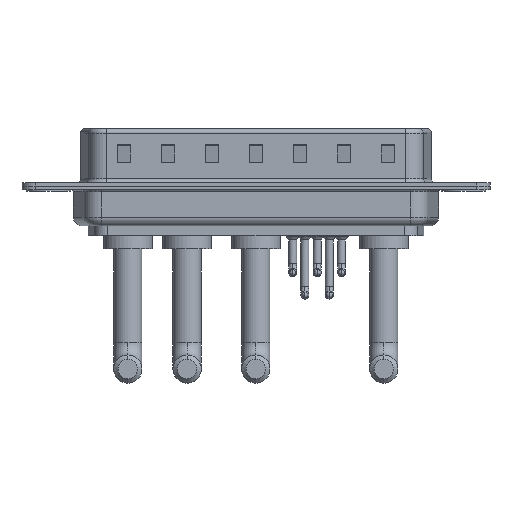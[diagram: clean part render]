
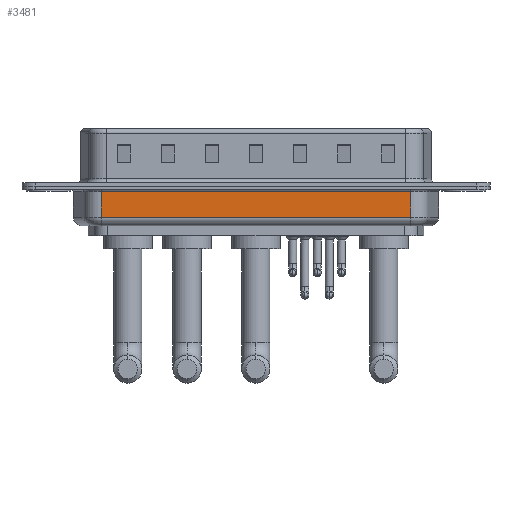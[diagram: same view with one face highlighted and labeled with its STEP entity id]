
A CAD part, front view. The second image highlights one B-rep face of the part: STEP entity #3481.
In plain terms, the highlighted planar face has unit normal (0, -1, 0).
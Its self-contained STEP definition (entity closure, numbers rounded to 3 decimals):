
#1218 = ORIENTED_EDGE ( 'NONE', *, *, #3673, .T. ) ;
#1629 = CARTESIAN_POINT ( 'NONE',  ( 6.006, -5.35, -4.5 ) ) ;
#1866 = VERTEX_POINT ( 'NONE', #13056 ) ;
#2395 = LINE ( 'NONE', #18587, #9191 ) ;
#3062 = ORIENTED_EDGE ( 'NONE', *, *, #18768, .F. ) ;
#3481 = ADVANCED_FACE ( 'NONE', ( #13874 ), #13770, .F. ) ;
#3673 = EDGE_CURVE ( 'NONE', #16897, #1866, #11369, .T. ) ;
#3857 = LINE ( 'NONE', #10237, #3866 ) ;
#3866 = VECTOR ( 'NONE', #16596, 1000. ) ;
#4992 = CARTESIAN_POINT ( 'NONE',  ( 6.006, -5.35, -3.5 ) ) ;
#6738 = CARTESIAN_POINT ( 'NONE',  ( 41.044, -5.35, -4.5 ) ) ;
#8534 = VERTEX_POINT ( 'NONE', #8943 ) ;
#8943 = CARTESIAN_POINT ( 'NONE',  ( 6.006, -5.35, -0.65 ) ) ;
#8949 = EDGE_CURVE ( 'NONE', #1866, #8534, #2395, .T. ) ;
#9097 = CARTESIAN_POINT ( 'NONE',  ( 41.044, -5.35, -3.5 ) ) ;
#9191 = VECTOR ( 'NONE', #15263, 1000. ) ;
#10237 = CARTESIAN_POINT ( 'NONE',  ( 6.006, -5.35, -3.5 ) ) ;
#11299 = AXIS2_PLACEMENT_3D ( 'NONE', #20211, #18664, #18765 ) ;
#11369 = LINE ( 'NONE', #6738, #12321 ) ;
#12321 = VECTOR ( 'NONE', #17715, 1000. ) ;
#12414 = EDGE_CURVE ( 'NONE', #15619, #16897, #3857, .T. ) ;
#12519 = ORIENTED_EDGE ( 'NONE', *, *, #8949, .T. ) ;
#13056 = CARTESIAN_POINT ( 'NONE',  ( 41.044, -5.35, -0.65 ) ) ;
#13770 = PLANE ( 'NONE',  #11299 ) ;
#13874 = FACE_OUTER_BOUND ( 'NONE', #20109, .T. ) ;
#15263 = DIRECTION ( 'NONE',  ( -1., 0., 0. ) ) ;
#15619 = VERTEX_POINT ( 'NONE', #4992 ) ;
#15856 = VECTOR ( 'NONE', #20639, 1000. ) ;
#15863 = LINE ( 'NONE', #1629, #15856 ) ;
#16035 = ORIENTED_EDGE ( 'NONE', *, *, #12414, .T. ) ;
#16596 = DIRECTION ( 'NONE',  ( 1., 0., 0. ) ) ;
#16897 = VERTEX_POINT ( 'NONE', #9097 ) ;
#17715 = DIRECTION ( 'NONE',  ( 0., 0., 1. ) ) ;
#18587 = CARTESIAN_POINT ( 'NONE',  ( 6.006, -5.35, -0.65 ) ) ;
#18664 = DIRECTION ( 'NONE',  ( 0., 1., 0. ) ) ;
#18765 = DIRECTION ( 'NONE',  ( 0., 0., 1. ) ) ;
#18768 = EDGE_CURVE ( 'NONE', #15619, #8534, #15863, .T. ) ;
#20109 = EDGE_LOOP ( 'NONE', ( #3062, #16035, #1218, #12519 ) ) ;
#20211 = CARTESIAN_POINT ( 'NONE',  ( 6.006, -5.35, -4.5 ) ) ;
#20639 = DIRECTION ( 'NONE',  ( 0., 0., 1. ) ) ;
